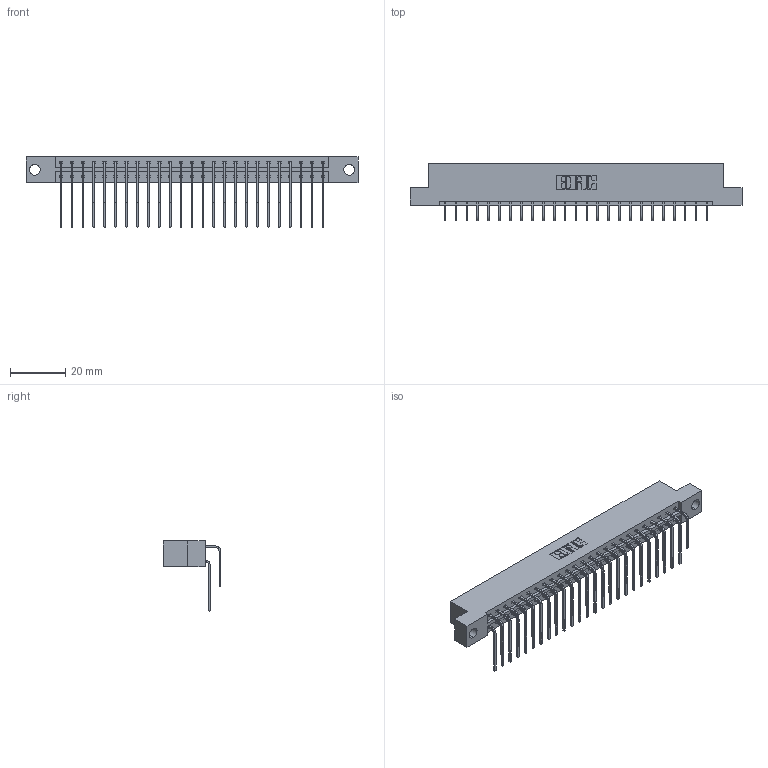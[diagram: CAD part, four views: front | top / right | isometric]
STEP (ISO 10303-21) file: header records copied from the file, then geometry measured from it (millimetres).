
FILE_DESCRIPTION (( 'STEP AP203' ), '1' );
FILE_NAME ('833-050-559-204.STEP', '2020-06-04T18:19:14', ( '' ), ( '' ), 'SwSTEP 2.0', 'SolidWorks 2020', '' );
FILE_SCHEMA (( 'CONFIG_CONTROL_DESIGN' ));
Length unit declared in the file: inch
Products named in the file (4): 345-292-001_558 559 Tail - 1; 833-050-559-204; 345-292-001_559 Tail - 2; 833 Part_Flush - .156 Dia - TH
Assembly tree (51 placements, depth 2):
  833-050-559-204
    833 Part_Flush - .156 Dia - TH
    345-292-001_558 559 Tail - 1  x25
    345-292-001_559 Tail - 2  x25
Bounding box: 120.6 x 20.9 x 25.53 mm (x, y, z)
Volume: 12354.1 mm3; surface area: 15659.1 mm2
Topology: 51 solids, 51 shells, 2814 faces, 8361 edges, 5506 vertices
Faces by surface type: plane 1970, cylinder 844
Entity records: 20069 total; most frequent: CARTESIAN_POINT 3397, ORIENTED_EDGE 3282, DIRECTION 2913, EDGE_CURVE 1641, LINE 1473, VECTOR 1473, VERTEX_POINT 1090, AXIS2_PLACEMENT_3D 720
